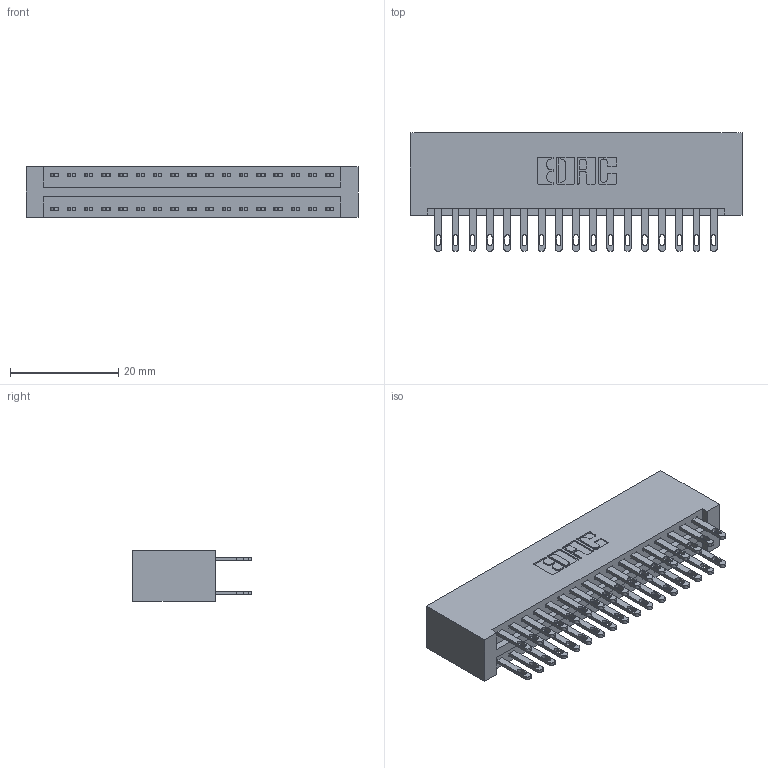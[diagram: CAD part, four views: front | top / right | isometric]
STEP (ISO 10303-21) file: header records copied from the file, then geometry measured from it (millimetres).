
FILE_DESCRIPTION (( 'STEP AP203' ), '1' );
FILE_NAME ('346-034-500-201.STEP', '2022-05-19T18:57:10', ( '' ), ( '' ), 'SwSTEP 2.0', 'SolidWorks 2020', '' );
FILE_SCHEMA (( 'CONFIG_CONTROL_DESIGN' ));
Length unit declared in the file: inch
Products named in the file (3): 346 Part_No Mounting Lugs; 345-292-001_345-293-100; 346-034-500-201
Assembly tree (35 placements, depth 2):
  346-034-500-201
    346 Part_No Mounting Lugs
    345-292-001_345-293-100  x34
Bounding box: 61.21 x 21.84 x 9.4 mm (x, y, z)
Volume: 6452.1 mm3; surface area: 8995 mm2
Topology: 35 solids, 35 shells, 1746 faces, 5303 edges, 3534 vertices
Faces by surface type: plane 1058, cylinder 688
Entity records: 14113 total; most frequent: CARTESIAN_POINT 2356, ORIENTED_EDGE 2290, DIRECTION 2125, EDGE_CURVE 1145, VECTOR 949, LINE 949, VERTEX_POINT 762, AXIS2_PLACEMENT_3D 588
